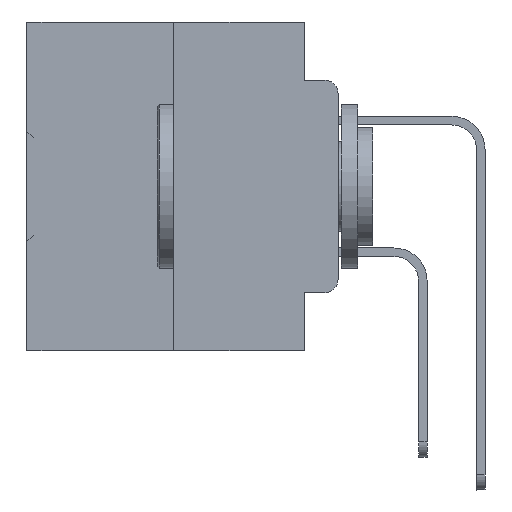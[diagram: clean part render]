
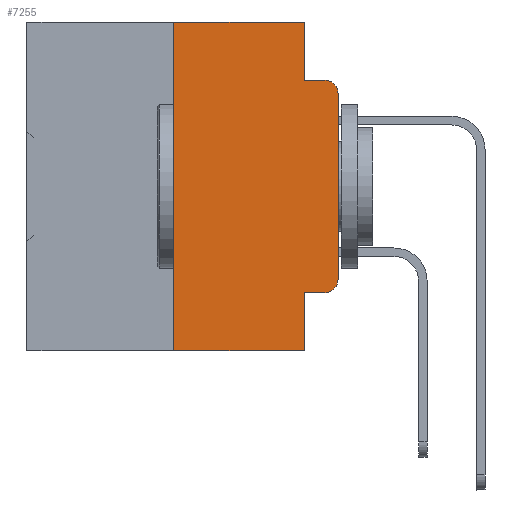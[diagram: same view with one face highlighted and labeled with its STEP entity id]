
A CAD part, left-side view. The second image highlights one B-rep face of the part: STEP entity #7255.
In plain terms, the highlighted planar face has unit normal (-1, 0, 0).
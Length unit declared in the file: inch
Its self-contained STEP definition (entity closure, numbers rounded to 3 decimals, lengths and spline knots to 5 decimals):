
#280 = LINE ( 'NONE', #8895, #30755 ) ;
#699 = AXIS2_PLACEMENT_3D ( 'NONE', #25214, #6386, #28368 ) ;
#857 = DIRECTION ( 'NONE',  ( 0., 0., -1. ) ) ;
#1334 = ORIENTED_EDGE ( 'NONE', *, *, #12883, .T. ) ;
#1615 = VECTOR ( 'NONE', #857, 39.37008 ) ;
#2599 = LINE ( 'NONE', #25907, #1615 ) ;
#2729 = VECTOR ( 'NONE', #25348, 39.37008 ) ;
#2802 = ORIENTED_EDGE ( 'NONE', *, *, #31801, .T. ) ;
#4654 = CARTESIAN_POINT ( 'NONE',  ( 0., 0., -0.1085 ) ) ;
#5105 = VERTEX_POINT ( 'NONE', #13955 ) ;
#5590 = AXIS2_PLACEMENT_3D ( 'NONE', #27657, #8832, #30764 ) ;
#5747 = DIRECTION ( 'NONE',  ( 0., 0., 1. ) ) ;
#5772 = ORIENTED_EDGE ( 'NONE', *, *, #23431, .F. ) ;
#6386 = DIRECTION ( 'NONE',  ( -1., 0., 0. ) ) ;
#6465 = CARTESIAN_POINT ( 'NONE',  ( 0., 0.25, 0. ) ) ;
#6627 = DIRECTION ( 'NONE',  ( 0., -1., 0. ) ) ;
#7153 = DIRECTION ( 'NONE',  ( 0., 0., 1. ) ) ;
#7255 = ADVANCED_FACE ( 'NONE', ( #40396 ), #14759, .F. ) ;
#7428 = CARTESIAN_POINT ( 'NONE',  ( 0., 0., -0.3915 ) ) ;
#8364 = CIRCLE ( 'NONE', #699, 0.02 ) ;
#8832 = DIRECTION ( 'NONE',  ( -1., 0., 0. ) ) ;
#8895 = CARTESIAN_POINT ( 'NONE',  ( 0., 0., 0. ) ) ;
#8916 = VERTEX_POINT ( 'NONE', #14020 ) ;
#9066 = CARTESIAN_POINT ( 'NONE',  ( 0., 0.473, -0.5 ) ) ;
#9441 = VECTOR ( 'NONE', #12731, 39.37008 ) ;
#9760 = CARTESIAN_POINT ( 'NONE',  ( 0., 0.051, -0.4115 ) ) ;
#10757 = EDGE_CURVE ( 'NONE', #32536, #11054, #12486, .T. ) ;
#10974 = CARTESIAN_POINT ( 'NONE',  ( 0., 0.02, -0.0885 ) ) ;
#11054 = VERTEX_POINT ( 'NONE', #7428 ) ;
#11060 = LINE ( 'NONE', #15863, #2729 ) ;
#12486 = CIRCLE ( 'NONE', #5590, 0.02 ) ;
#12731 = DIRECTION ( 'NONE',  ( 0., -1., 0. ) ) ;
#12883 = EDGE_CURVE ( 'NONE', #39614, #32536, #25597, .T. ) ;
#13492 = CARTESIAN_POINT ( 'NONE',  ( 0., 0.25, 0. ) ) ;
#13955 = CARTESIAN_POINT ( 'NONE',  ( 0., 0.051, 0. ) ) ;
#14020 = CARTESIAN_POINT ( 'NONE',  ( 0., 0.25, -0.5 ) ) ;
#14431 = CARTESIAN_POINT ( 'NONE',  ( 0., 0.051, 0. ) ) ;
#14759 = PLANE ( 'NONE',  #33878 ) ;
#15516 = DIRECTION ( 'NONE',  ( 0., -1., 0. ) ) ;
#15863 = CARTESIAN_POINT ( 'NONE',  ( 0., 0.473, 0. ) ) ;
#15988 = CARTESIAN_POINT ( 'NONE',  ( 0., 0.02, -0.4115 ) ) ;
#16831 = LINE ( 'NONE', #31508, #9441 ) ;
#17077 = ORIENTED_EDGE ( 'NONE', *, *, #19796, .T. ) ;
#17908 = CARTESIAN_POINT ( 'NONE',  ( 0., 0.473, 0. ) ) ;
#18652 = EDGE_LOOP ( 'NONE', ( #2802, #21509, #29818, #5772, #23461, #40083, #17077, #25438, #1334, #27414 ) ) ;
#19248 = EDGE_CURVE ( 'NONE', #39614, #38692, #2599, .T. ) ;
#19796 = EDGE_CURVE ( 'NONE', #8916, #38692, #31020, .T. ) ;
#20751 = CARTESIAN_POINT ( 'NONE',  ( 0., 0.051, -0.5 ) ) ;
#21087 = DIRECTION ( 'NONE',  ( 0., 0., -1. ) ) ;
#21174 = VECTOR ( 'NONE', #7153, 39.37008 ) ;
#21349 = EDGE_CURVE ( 'NONE', #8916, #35910, #37823, .T. ) ;
#21509 = ORIENTED_EDGE ( 'NONE', *, *, #29719, .T. ) ;
#21991 = VERTEX_POINT ( 'NONE', #4654 ) ;
#22707 = VECTOR ( 'NONE', #15516, 39.37008 ) ;
#23431 = EDGE_CURVE ( 'NONE', #5105, #35663, #28821, .T. ) ;
#23461 = ORIENTED_EDGE ( 'NONE', *, *, #37123, .F. ) ;
#24584 = VECTOR ( 'NONE', #6627, 39.37008 ) ;
#25214 = CARTESIAN_POINT ( 'NONE',  ( 0., 0.02, -0.1085 ) ) ;
#25336 = CARTESIAN_POINT ( 'NONE',  ( 0., 0.051, -0.4115 ) ) ;
#25348 = DIRECTION ( 'NONE',  ( 0., -1., 0. ) ) ;
#25438 = ORIENTED_EDGE ( 'NONE', *, *, #19248, .F. ) ;
#25597 = LINE ( 'NONE', #9760, #24584 ) ;
#25907 = CARTESIAN_POINT ( 'NONE',  ( 0., 0.051, 0. ) ) ;
#27055 = DIRECTION ( 'NONE',  ( 0., 0., -1. ) ) ;
#27414 = ORIENTED_EDGE ( 'NONE', *, *, #10757, .T. ) ;
#27635 = EDGE_CURVE ( 'NONE', #35663, #28823, #16831, .T. ) ;
#27657 = CARTESIAN_POINT ( 'NONE',  ( 0., 0.02, -0.3915 ) ) ;
#27850 = VECTOR ( 'NONE', #27055, 39.37008 ) ;
#28368 = DIRECTION ( 'NONE',  ( 0., 0., -1. ) ) ;
#28821 = LINE ( 'NONE', #14431, #27850 ) ;
#28823 = VERTEX_POINT ( 'NONE', #10974 ) ;
#29719 = EDGE_CURVE ( 'NONE', #21991, #28823, #8364, .T. ) ;
#29818 = ORIENTED_EDGE ( 'NONE', *, *, #27635, .F. ) ;
#30346 = CARTESIAN_POINT ( 'NONE',  ( 0., 0.051, -0.0885 ) ) ;
#30755 = VECTOR ( 'NONE', #5747, 39.37008 ) ;
#30764 = DIRECTION ( 'NONE',  ( 0., 0., -1. ) ) ;
#31020 = LINE ( 'NONE', #9066, #22707 ) ;
#31508 = CARTESIAN_POINT ( 'NONE',  ( 0., 0.051, -0.0885 ) ) ;
#31801 = EDGE_CURVE ( 'NONE', #11054, #21991, #280, .T. ) ;
#32536 = VERTEX_POINT ( 'NONE', #15988 ) ;
#33878 = AXIS2_PLACEMENT_3D ( 'NONE', #17908, #39794, #21087 ) ;
#35663 = VERTEX_POINT ( 'NONE', #30346 ) ;
#35910 = VERTEX_POINT ( 'NONE', #6465 ) ;
#37123 = EDGE_CURVE ( 'NONE', #35910, #5105, #11060, .T. ) ;
#37823 = LINE ( 'NONE', #13492, #21174 ) ;
#38692 = VERTEX_POINT ( 'NONE', #20751 ) ;
#39614 = VERTEX_POINT ( 'NONE', #25336 ) ;
#39794 = DIRECTION ( 'NONE',  ( 1., 0., 0. ) ) ;
#40083 = ORIENTED_EDGE ( 'NONE', *, *, #21349, .F. ) ;
#40396 = FACE_OUTER_BOUND ( 'NONE', #18652, .T. ) ;
